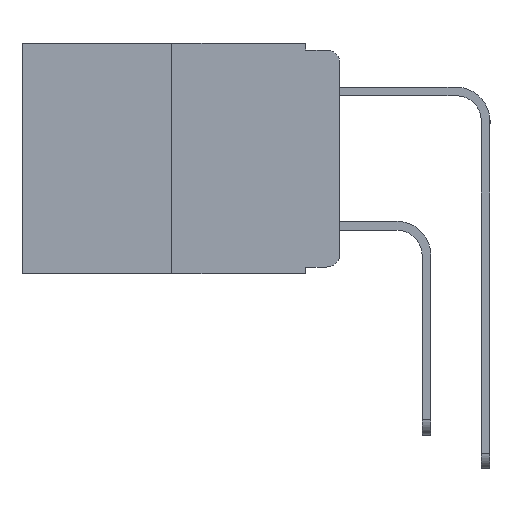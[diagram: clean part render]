
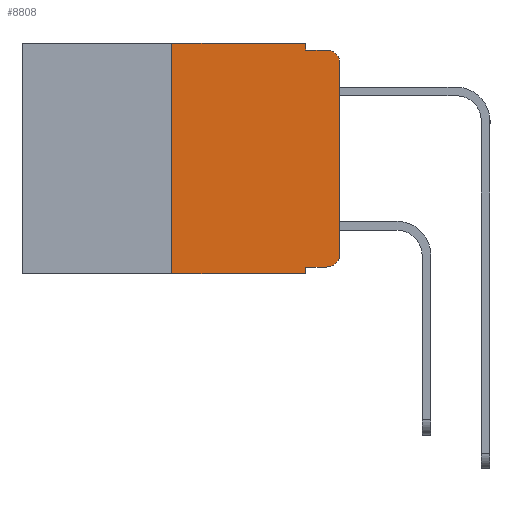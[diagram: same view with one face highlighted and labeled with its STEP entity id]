
A CAD part, left-side view. The second image highlights one B-rep face of the part: STEP entity #8808.
In plain terms, the highlighted planar face has unit normal (-1, 0, 0).
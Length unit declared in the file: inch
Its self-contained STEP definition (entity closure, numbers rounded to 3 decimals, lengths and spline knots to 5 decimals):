
#240 = CARTESIAN_POINT ( 'NONE',  ( 0., 0.25, 0. ) ) ;
#570 = VECTOR ( 'NONE', #1244, 39.37008 ) ;
#654 = VERTEX_POINT ( 'NONE', #13784 ) ;
#782 = CARTESIAN_POINT ( 'NONE',  ( 0., 0.473, -0.343 ) ) ;
#799 = ORIENTED_EDGE ( 'NONE', *, *, #5119, .T. ) ;
#1056 = VERTEX_POINT ( 'NONE', #11319 ) ;
#1112 = CIRCLE ( 'NONE', #9037, 0.02 ) ;
#1244 = DIRECTION ( 'NONE',  ( 0., 0., -1. ) ) ;
#1853 = CARTESIAN_POINT ( 'NONE',  ( 0., 0.02, -0.01 ) ) ;
#1901 = CARTESIAN_POINT ( 'NONE',  ( 0., 0.02, -0.03 ) ) ;
#1940 = LINE ( 'NONE', #5108, #7929 ) ;
#1964 = VERTEX_POINT ( 'NONE', #7715 ) ;
#2000 = VECTOR ( 'NONE', #4494, 39.37008 ) ;
#2249 = VERTEX_POINT ( 'NONE', #13404 ) ;
#2290 = LINE ( 'NONE', #16235, #6096 ) ;
#2641 = EDGE_CURVE ( 'NONE', #3581, #5630, #2290, .T. ) ;
#2668 = ORIENTED_EDGE ( 'NONE', *, *, #9091, .T. ) ;
#2911 = CARTESIAN_POINT ( 'NONE',  ( 0., 0.051, 0. ) ) ;
#3062 = DIRECTION ( 'NONE',  ( 1., 0., 0. ) ) ;
#3190 = DIRECTION ( 'NONE',  ( 0., 0., -1. ) ) ;
#3254 = ORIENTED_EDGE ( 'NONE', *, *, #12993, .T. ) ;
#3287 = ORIENTED_EDGE ( 'NONE', *, *, #6913, .F. ) ;
#3326 = CARTESIAN_POINT ( 'NONE',  ( 0., 0.02, -0.313 ) ) ;
#3489 = EDGE_CURVE ( 'NONE', #5630, #1964, #5085, .T. ) ;
#3507 = CIRCLE ( 'NONE', #14427, 0.02 ) ;
#3581 = VERTEX_POINT ( 'NONE', #7503 ) ;
#3939 = CARTESIAN_POINT ( 'NONE',  ( 0., 0.051, -0.333 ) ) ;
#4151 = VERTEX_POINT ( 'NONE', #3939 ) ;
#4255 = CARTESIAN_POINT ( 'NONE',  ( 0., 0.473, 0. ) ) ;
#4270 = ORIENTED_EDGE ( 'NONE', *, *, #9205, .F. ) ;
#4494 = DIRECTION ( 'NONE',  ( 0., -1., 0. ) ) ;
#4616 = DIRECTION ( 'NONE',  ( 0., 0., -1. ) ) ;
#4903 = ORIENTED_EDGE ( 'NONE', *, *, #3489, .F. ) ;
#5085 = LINE ( 'NONE', #4255, #10321 ) ;
#5108 = CARTESIAN_POINT ( 'NONE',  ( 0., 0.051, -0.01 ) ) ;
#5119 = EDGE_CURVE ( 'NONE', #4151, #7198, #12264, .T. ) ;
#5220 = DIRECTION ( 'NONE',  ( 0., -1., 0. ) ) ;
#5444 = VERTEX_POINT ( 'NONE', #11897 ) ;
#5470 = ORIENTED_EDGE ( 'NONE', *, *, #2641, .F. ) ;
#5610 = VECTOR ( 'NONE', #8765, 39.37008 ) ;
#5630 = VERTEX_POINT ( 'NONE', #240 ) ;
#5675 = ORIENTED_EDGE ( 'NONE', *, *, #14958, .T. ) ;
#6096 = VECTOR ( 'NONE', #11220, 39.37008 ) ;
#6513 = CARTESIAN_POINT ( 'NONE',  ( 0., 0.051, -0.333 ) ) ;
#6552 = VERTEX_POINT ( 'NONE', #1853 ) ;
#6913 = EDGE_CURVE ( 'NONE', #654, #6552, #1940, .T. ) ;
#7002 = LINE ( 'NONE', #7623, #570 ) ;
#7198 = VERTEX_POINT ( 'NONE', #13369 ) ;
#7320 = ORIENTED_EDGE ( 'NONE', *, *, #12894, .F. ) ;
#7503 = CARTESIAN_POINT ( 'NONE',  ( 0., 0.25, -0.343 ) ) ;
#7623 = CARTESIAN_POINT ( 'NONE',  ( 0., 0.051, 0. ) ) ;
#7715 = CARTESIAN_POINT ( 'NONE',  ( 0., 0.051, 0. ) ) ;
#7929 = VECTOR ( 'NONE', #8912, 39.37008 ) ;
#8619 = LINE ( 'NONE', #16391, #5610 ) ;
#8765 = DIRECTION ( 'NONE',  ( 0., 0., 1. ) ) ;
#8808 = ADVANCED_FACE ( 'NONE', ( #10069 ), #10772, .F. ) ;
#8912 = DIRECTION ( 'NONE',  ( 0., -1., 0. ) ) ;
#9037 = AXIS2_PLACEMENT_3D ( 'NONE', #3326, #12326, #4616 ) ;
#9091 = EDGE_CURVE ( 'NONE', #5444, #2249, #8619, .T. ) ;
#9149 = VECTOR ( 'NONE', #9800, 39.37008 ) ;
#9205 = EDGE_CURVE ( 'NONE', #1964, #654, #7002, .T. ) ;
#9467 = CARTESIAN_POINT ( 'NONE',  ( 0., 0.473, 0. ) ) ;
#9800 = DIRECTION ( 'NONE',  ( 0., -1., 0. ) ) ;
#10069 = FACE_OUTER_BOUND ( 'NONE', #12939, .T. ) ;
#10321 = VECTOR ( 'NONE', #5220, 39.37008 ) ;
#10690 = DIRECTION ( 'NONE',  ( 0., 0., -1. ) ) ;
#10772 = PLANE ( 'NONE',  #14677 ) ;
#10896 = DIRECTION ( 'NONE',  ( -1., 0., 0. ) ) ;
#11220 = DIRECTION ( 'NONE',  ( 0., 0., 1. ) ) ;
#11319 = CARTESIAN_POINT ( 'NONE',  ( 0., 0.051, -0.343 ) ) ;
#11573 = VECTOR ( 'NONE', #10690, 39.37008 ) ;
#11897 = CARTESIAN_POINT ( 'NONE',  ( 0., 0., -0.313 ) ) ;
#12058 = DIRECTION ( 'NONE',  ( 0., 0., -1. ) ) ;
#12168 = LINE ( 'NONE', #782, #9149 ) ;
#12249 = ORIENTED_EDGE ( 'NONE', *, *, #12441, .T. ) ;
#12264 = LINE ( 'NONE', #6513, #2000 ) ;
#12326 = DIRECTION ( 'NONE',  ( -1., 0., 0. ) ) ;
#12441 = EDGE_CURVE ( 'NONE', #7198, #5444, #1112, .T. ) ;
#12894 = EDGE_CURVE ( 'NONE', #4151, #1056, #15710, .T. ) ;
#12939 = EDGE_LOOP ( 'NONE', ( #2668, #3254, #3287, #4270, #4903, #5470, #5675, #7320, #799, #12249 ) ) ;
#12993 = EDGE_CURVE ( 'NONE', #2249, #6552, #3507, .T. ) ;
#13369 = CARTESIAN_POINT ( 'NONE',  ( 0., 0.02, -0.333 ) ) ;
#13404 = CARTESIAN_POINT ( 'NONE',  ( 0., 0., -0.03 ) ) ;
#13784 = CARTESIAN_POINT ( 'NONE',  ( 0., 0.051, -0.01 ) ) ;
#14427 = AXIS2_PLACEMENT_3D ( 'NONE', #1901, #10896, #3190 ) ;
#14677 = AXIS2_PLACEMENT_3D ( 'NONE', #9467, #3062, #12058 ) ;
#14958 = EDGE_CURVE ( 'NONE', #3581, #1056, #12168, .T. ) ;
#15710 = LINE ( 'NONE', #2911, #11573 ) ;
#16235 = CARTESIAN_POINT ( 'NONE',  ( 0., 0.25, 0. ) ) ;
#16391 = CARTESIAN_POINT ( 'NONE',  ( 0., 0., 0. ) ) ;
